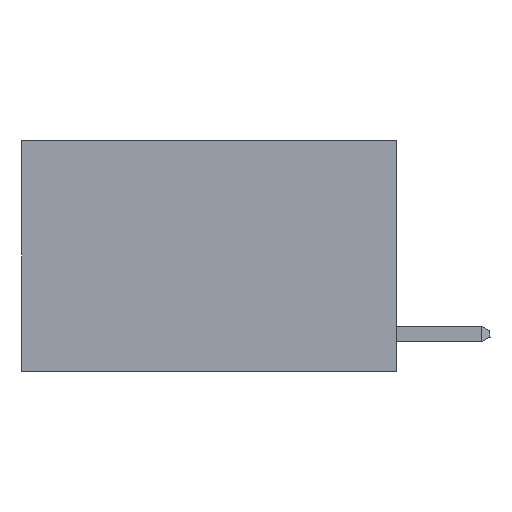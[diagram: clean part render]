
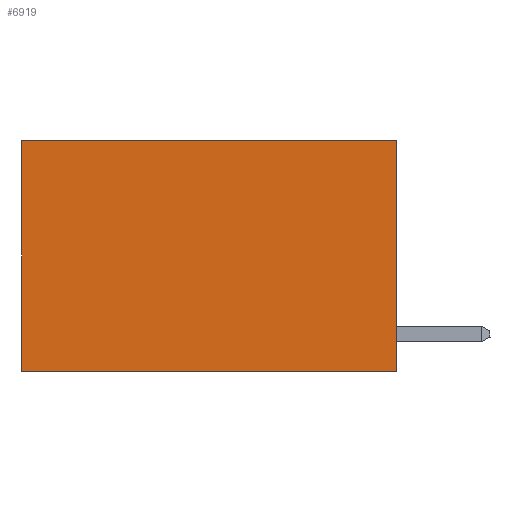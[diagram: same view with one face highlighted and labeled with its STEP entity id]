
A CAD part, left-side view. The second image highlights one B-rep face of the part: STEP entity #6919.
In plain terms, the highlighted planar face has unit normal (-1, 0, 0).
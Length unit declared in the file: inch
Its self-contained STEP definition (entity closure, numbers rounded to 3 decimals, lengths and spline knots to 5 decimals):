
#32 = ORIENTED_EDGE ( 'NONE', *, *, #2599, .T. ) ;
#89 = CARTESIAN_POINT ( 'NONE',  ( 0.2625, 0., -0.37 ) ) ;
#194 = EDGE_CURVE ( 'NONE', #2526, #364, #6388, .T. ) ;
#364 = VERTEX_POINT ( 'NONE', #2934 ) ;
#614 = PLANE ( 'NONE',  #7848 ) ;
#633 = ORIENTED_EDGE ( 'NONE', *, *, #8436, .F. ) ;
#951 = VECTOR ( 'NONE', #9203, 39.37008 ) ;
#1175 = DIRECTION ( 'NONE',  ( 0., 1., 0. ) ) ;
#1632 = CARTESIAN_POINT ( 'NONE',  ( 0.2625, 0., 0. ) ) ;
#1689 = ORIENTED_EDGE ( 'NONE', *, *, #194, .F. ) ;
#2459 = LINE ( 'NONE', #9369, #951 ) ;
#2526 = VERTEX_POINT ( 'NONE', #7228 ) ;
#2558 = VECTOR ( 'NONE', #4234, 39.37008 ) ;
#2599 = EDGE_CURVE ( 'NONE', #7113, #364, #2459, .T. ) ;
#2934 = CARTESIAN_POINT ( 'NONE',  ( 0.2625, 0.6, -0.37 ) ) ;
#3021 = ORIENTED_EDGE ( 'NONE', *, *, #3382, .T. ) ;
#3169 = LINE ( 'NONE', #6669, #4634 ) ;
#3382 = EDGE_CURVE ( 'NONE', #9941, #7113, #3169, .T. ) ;
#3931 = DIRECTION ( 'NONE',  ( 0., 1., 0. ) ) ;
#4111 = DIRECTION ( 'NONE',  ( 0., 0., -1. ) ) ;
#4234 = DIRECTION ( 'NONE',  ( 0., 0., -1. ) ) ;
#4268 = EDGE_LOOP ( 'NONE', ( #32, #1689, #633, #3021 ) ) ;
#4634 = VECTOR ( 'NONE', #3931, 39.37008 ) ;
#5644 = DIRECTION ( 'NONE',  ( 1., 0., 0. ) ) ;
#6388 = LINE ( 'NONE', #89, #8291 ) ;
#6669 = CARTESIAN_POINT ( 'NONE',  ( 0.2625, 0., 0. ) ) ;
#6919 = ADVANCED_FACE ( 'NONE', ( #7561 ), #614, .F. ) ;
#7038 = LINE ( 'NONE', #1632, #2558 ) ;
#7113 = VERTEX_POINT ( 'NONE', #7957 ) ;
#7228 = CARTESIAN_POINT ( 'NONE',  ( 0.2625, 0., -0.37 ) ) ;
#7561 = FACE_OUTER_BOUND ( 'NONE', #4268, .T. ) ;
#7848 = AXIS2_PLACEMENT_3D ( 'NONE', #10113, #5644, #4111 ) ;
#7957 = CARTESIAN_POINT ( 'NONE',  ( 0.2625, 0.6, 0. ) ) ;
#8291 = VECTOR ( 'NONE', #1175, 39.37008 ) ;
#8436 = EDGE_CURVE ( 'NONE', #9941, #2526, #7038, .T. ) ;
#9203 = DIRECTION ( 'NONE',  ( 0., 0., -1. ) ) ;
#9369 = CARTESIAN_POINT ( 'NONE',  ( 0.2625, 0.6, 0. ) ) ;
#9850 = CARTESIAN_POINT ( 'NONE',  ( 0.2625, 0., 0. ) ) ;
#9941 = VERTEX_POINT ( 'NONE', #9850 ) ;
#10113 = CARTESIAN_POINT ( 'NONE',  ( 0.2625, 0., 0. ) ) ;
